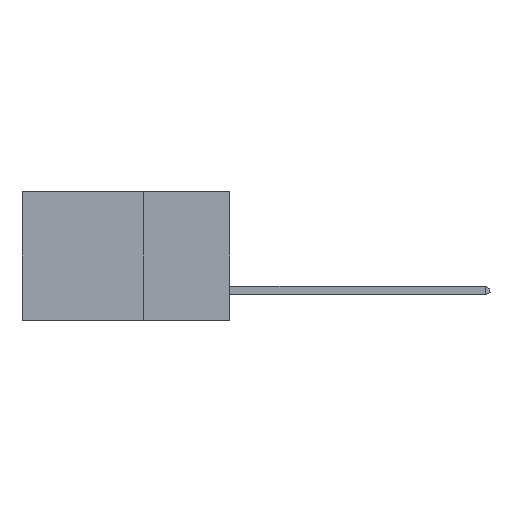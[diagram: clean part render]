
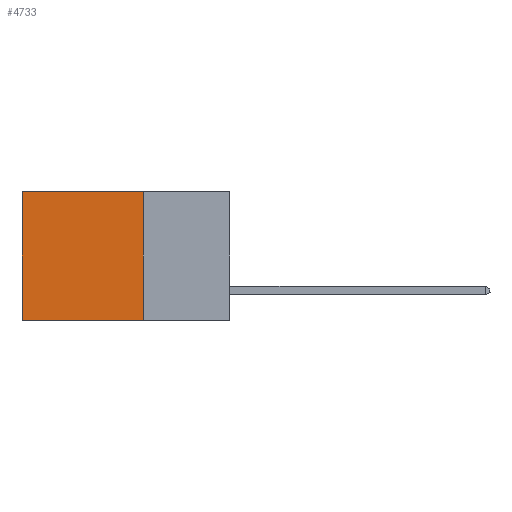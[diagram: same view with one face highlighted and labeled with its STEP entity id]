
A CAD part, left-side view. The second image highlights one B-rep face of the part: STEP entity #4733.
In plain terms, the highlighted planar face has unit normal (-1, 0, 0).
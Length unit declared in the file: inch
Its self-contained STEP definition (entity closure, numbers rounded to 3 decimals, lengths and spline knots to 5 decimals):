
#12 = ORIENTED_EDGE ( 'NONE', *, *, #531, .F. ) ;
#96 = VERTEX_POINT ( 'NONE', #18977 ) ;
#531 = EDGE_CURVE ( 'NONE', #22529, #96, #2493, .T. ) ;
#849 = ORIENTED_EDGE ( 'NONE', *, *, #16693, .F. ) ;
#1780 = DIRECTION ( 'NONE',  ( 0., 0., -1. ) ) ;
#2493 = LINE ( 'NONE', #19260, #13995 ) ;
#3666 = LINE ( 'NONE', #11402, #13394 ) ;
#4733 = ADVANCED_FACE ( 'NONE', ( #14494 ), #11356, .F. ) ;
#5274 = VERTEX_POINT ( 'NONE', #7421 ) ;
#5349 = LINE ( 'NONE', #21005, #11751 ) ;
#5430 = DIRECTION ( 'NONE',  ( 1., 0., 0. ) ) ;
#5914 = LINE ( 'NONE', #13295, #24206 ) ;
#5977 = ORIENTED_EDGE ( 'NONE', *, *, #15208, .T. ) ;
#7421 = CARTESIAN_POINT ( 'NONE',  ( 0.298, 0.6, -0.37 ) ) ;
#9427 = CARTESIAN_POINT ( 'NONE',  ( 0.298, 0.6, 0. ) ) ;
#9496 = CARTESIAN_POINT ( 'NONE',  ( 0.298, 0.25, 0. ) ) ;
#10979 = AXIS2_PLACEMENT_3D ( 'NONE', #9496, #5430, #1780 ) ;
#11356 = PLANE ( 'NONE',  #10979 ) ;
#11402 = CARTESIAN_POINT ( 'NONE',  ( 0.298, 0.25, -0.37 ) ) ;
#11571 = DIRECTION ( 'NONE',  ( 0., 0., -1. ) ) ;
#11751 = VECTOR ( 'NONE', #11571, 39.37008 ) ;
#11772 = CARTESIAN_POINT ( 'NONE',  ( 0.298, 0.25, 0. ) ) ;
#12741 = VERTEX_POINT ( 'NONE', #9427 ) ;
#13211 = DIRECTION ( 'NONE',  ( 0., 1., 0. ) ) ;
#13295 = CARTESIAN_POINT ( 'NONE',  ( 0.298, 0.25, 0. ) ) ;
#13394 = VECTOR ( 'NONE', #15333, 39.37008 ) ;
#13995 = VECTOR ( 'NONE', #21109, 39.37008 ) ;
#14494 = FACE_OUTER_BOUND ( 'NONE', #14701, .T. ) ;
#14701 = EDGE_LOOP ( 'NONE', ( #5977, #849, #12, #16188 ) ) ;
#15208 = EDGE_CURVE ( 'NONE', #12741, #5274, #5349, .T. ) ;
#15333 = DIRECTION ( 'NONE',  ( 0., 1., 0. ) ) ;
#16188 = ORIENTED_EDGE ( 'NONE', *, *, #20520, .T. ) ;
#16693 = EDGE_CURVE ( 'NONE', #96, #5274, #3666, .T. ) ;
#18977 = CARTESIAN_POINT ( 'NONE',  ( 0.298, 0.25, -0.37 ) ) ;
#19260 = CARTESIAN_POINT ( 'NONE',  ( 0.298, 0.25, 0. ) ) ;
#20520 = EDGE_CURVE ( 'NONE', #22529, #12741, #5914, .T. ) ;
#21005 = CARTESIAN_POINT ( 'NONE',  ( 0.298, 0.6, 0. ) ) ;
#21109 = DIRECTION ( 'NONE',  ( 0., 0., -1. ) ) ;
#22529 = VERTEX_POINT ( 'NONE', #11772 ) ;
#24206 = VECTOR ( 'NONE', #13211, 39.37008 ) ;
